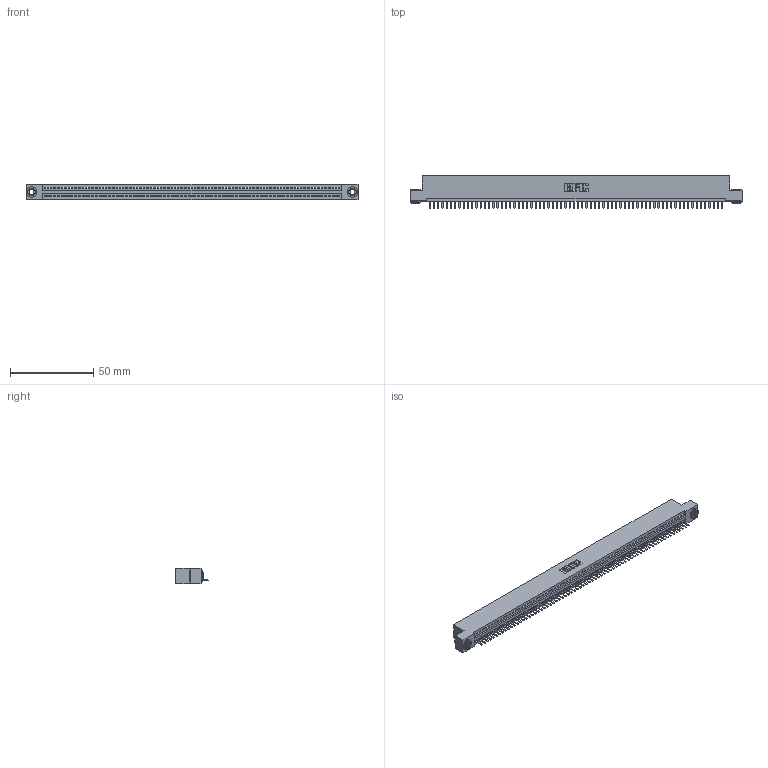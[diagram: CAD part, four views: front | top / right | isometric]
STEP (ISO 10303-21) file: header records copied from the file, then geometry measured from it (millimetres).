
FILE_DESCRIPTION (( 'STEP AP203' ), '1' );
FILE_NAME ('345-070-520-103.STEP', '2019-10-12T14:31:51', ( '' ), ( '' ), 'SwSTEP 2.0', 'SolidWorks 2016', '' );
FILE_SCHEMA (( 'CONFIG_CONTROL_DESIGN' ));
Length unit declared in the file: inch
Products named in the file (4): 345-292-001_345-293-120; 345-250-002_345-250-002-102; 345-070-520-103; 345 Part_Flush Mounting Lugs - 0.156 Dia-TH
Assembly tree (73 placements, depth 2):
  345-070-520-103
    345 Part_Flush Mounting Lugs - 0.156 Dia-TH
    345-292-001_345-293-120  x70
    345-250-002_345-250-002-102  x2
Bounding box: 199.01 x 19.68 x 9.4 mm (x, y, z)
Volume: 18949.5 mm3; surface area: 25118.4 mm2
Topology: 73 solids, 73 shells, 4504 faces, 13297 edges, 8674 vertices
Faces by surface type: plane 3030, cylinder 1466, cone 8
Entity records: 49678 total; most frequent: CARTESIAN_POINT 8593, ORIENTED_EDGE 8578, DIRECTION 7483, EDGE_CURVE 4289, VECTOR 3849, LINE 3849, VERTEX_POINT 2854, AXIS2_PLACEMENT_3D 1817
